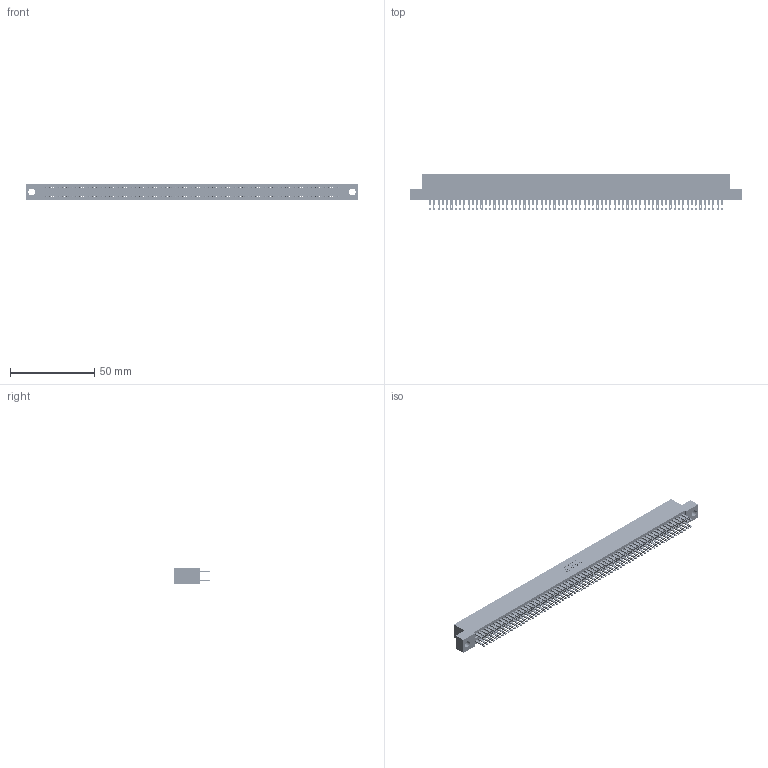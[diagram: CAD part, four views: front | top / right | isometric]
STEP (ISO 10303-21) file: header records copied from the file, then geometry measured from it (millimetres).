
FILE_DESCRIPTION (( 'STEP AP203' ), '1' );
FILE_NAME ('345-138-500-204.STEP', '2021-05-25T23:42:08', ( '' ), ( '' ), 'SwSTEP 2.0', 'SolidWorks 2020', '' );
FILE_SCHEMA (( 'CONFIG_CONTROL_DESIGN' ));
Length unit declared in the file: inch
Products named in the file (3): 345 Part_Flush Mounting Lugs - 0.156 Dia-TI; 345-138-500-204; 345-292-001_345-293-100
Assembly tree (139 placements, depth 2):
  345-138-500-204
    345 Part_Flush Mounting Lugs - 0.156 Dia-TI
    345-292-001_345-293-100  x138
Bounding box: 196.47 x 21.51 x 9.4 mm (x, y, z)
Volume: 19651.6 mm3; surface area: 30830.4 mm2
Topology: 139 solids, 139 shells, 6488 faces, 19835 edges, 13222 vertices
Faces by surface type: plane 3820, cylinder 2668
Entity records: 50853 total; most frequent: CARTESIAN_POINT 8502, ORIENTED_EDGE 8434, DIRECTION 7465, EDGE_CURVE 4217, LINE 3805, VECTOR 3805, VERTEX_POINT 2810, AXIS2_PLACEMENT_3D 1830
